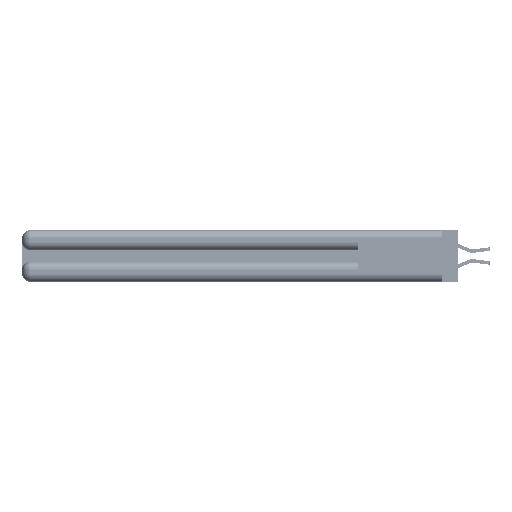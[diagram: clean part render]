
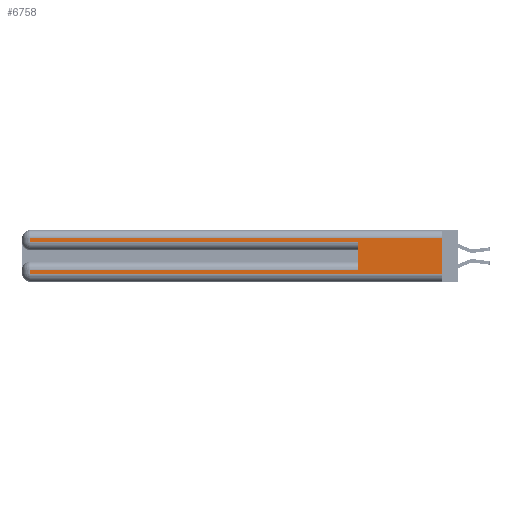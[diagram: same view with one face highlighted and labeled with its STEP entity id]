
A CAD part, left-side view. The second image highlights one B-rep face of the part: STEP entity #6758.
In plain terms, the highlighted planar face has unit normal (-1, 0, 0).
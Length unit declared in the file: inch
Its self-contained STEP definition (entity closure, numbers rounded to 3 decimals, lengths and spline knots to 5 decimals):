
#1256 = LINE ( 'NONE', #49349, #53000 ) ;
#1796 = VERTEX_POINT ( 'NONE', #38416 ) ;
#1999 = CARTESIAN_POINT ( 'NONE',  ( 0., 0., 0.37 ) ) ;
#2927 = ORIENTED_EDGE ( 'NONE', *, *, #8571, .T. ) ;
#2990 = EDGE_CURVE ( 'NONE', #17240, #33682, #16627, .T. ) ;
#3101 = VECTOR ( 'NONE', #3349, 39.37008 ) ;
#3349 = DIRECTION ( 'NONE',  ( 0., -1., 0. ) ) ;
#3509 = CARTESIAN_POINT ( 'NONE',  ( 0., 0., 0.285 ) ) ;
#3828 = DIRECTION ( 'NONE',  ( 0., 1., 0. ) ) ;
#4285 = LINE ( 'NONE', #1999, #22277 ) ;
#6686 = DIRECTION ( 'NONE',  ( 0., 0., -1. ) ) ;
#6758 = ADVANCED_FACE ( 'NONE', ( #38635 ), #25982, .F. ) ;
#7162 = CARTESIAN_POINT ( 'NONE',  ( 0., 0., 0.31 ) ) ;
#8322 = EDGE_CURVE ( 'NONE', #31892, #1796, #20441, .T. ) ;
#8571 = EDGE_CURVE ( 'NONE', #39538, #28233, #33320, .T. ) ;
#9520 = VECTOR ( 'NONE', #6686, 39.37008 ) ;
#10429 = CARTESIAN_POINT ( 'NONE',  ( 0., 2.94, 0.31 ) ) ;
#10934 = EDGE_CURVE ( 'NONE', #31908, #1796, #4285, .T. ) ;
#11728 = DIRECTION ( 'NONE',  ( 0., -1., 0. ) ) ;
#12403 = ORIENTED_EDGE ( 'NONE', *, *, #24803, .T. ) ;
#13508 = CARTESIAN_POINT ( 'NONE',  ( 0., 0., 0.37 ) ) ;
#14196 = DIRECTION ( 'NONE',  ( 0., 0., -1. ) ) ;
#16627 = LINE ( 'NONE', #38721, #38555 ) ;
#17240 = VERTEX_POINT ( 'NONE', #43411 ) ;
#18455 = EDGE_CURVE ( 'NONE', #31908, #39538, #1256, .T. ) ;
#19855 = CARTESIAN_POINT ( 'NONE',  ( 0., 0., 0.06 ) ) ;
#20441 = LINE ( 'NONE', #19855, #3101 ) ;
#20794 = CARTESIAN_POINT ( 'NONE',  ( 0., 2.94, 0.285 ) ) ;
#21279 = VECTOR ( 'NONE', #11728, 39.37008 ) ;
#21494 = DIRECTION ( 'NONE',  ( 0., 0., 1. ) ) ;
#22235 = AXIS2_PLACEMENT_3D ( 'NONE', #13508, #42412, #46280 ) ;
#22277 = VECTOR ( 'NONE', #14196, 39.37008 ) ;
#23624 = CARTESIAN_POINT ( 'NONE',  ( 0., 2.94, 0.37 ) ) ;
#23753 = VERTEX_POINT ( 'NONE', #45072 ) ;
#24803 = EDGE_CURVE ( 'NONE', #33682, #31892, #35378, .T. ) ;
#25114 = ORIENTED_EDGE ( 'NONE', *, *, #2990, .T. ) ;
#25233 = LINE ( 'NONE', #3509, #21279 ) ;
#25982 = PLANE ( 'NONE',  #22235 ) ;
#26838 = ORIENTED_EDGE ( 'NONE', *, *, #38016, .F. ) ;
#27167 = LINE ( 'NONE', #29460, #42038 ) ;
#28233 = VERTEX_POINT ( 'NONE', #20794 ) ;
#29460 = CARTESIAN_POINT ( 'NONE',  ( 0., 0.6, 0.145 ) ) ;
#31892 = VERTEX_POINT ( 'NONE', #52758 ) ;
#31908 = VERTEX_POINT ( 'NONE', #7162 ) ;
#33320 = LINE ( 'NONE', #23624, #9520 ) ;
#33519 = ORIENTED_EDGE ( 'NONE', *, *, #8322, .T. ) ;
#33682 = VERTEX_POINT ( 'NONE', #35364 ) ;
#35171 = CARTESIAN_POINT ( 'NONE',  ( 0., 2.94, 0.37 ) ) ;
#35364 = CARTESIAN_POINT ( 'NONE',  ( 0., 2.94, 0.085 ) ) ;
#35378 = LINE ( 'NONE', #35171, #38596 ) ;
#35699 = ORIENTED_EDGE ( 'NONE', *, *, #10934, .F. ) ;
#38016 = EDGE_CURVE ( 'NONE', #17240, #23753, #27167, .T. ) ;
#38258 = ORIENTED_EDGE ( 'NONE', *, *, #18455, .T. ) ;
#38358 = DIRECTION ( 'NONE',  ( 0., 1., 0. ) ) ;
#38397 = EDGE_CURVE ( 'NONE', #28233, #23753, #25233, .T. ) ;
#38416 = CARTESIAN_POINT ( 'NONE',  ( 0., 0., 0.06 ) ) ;
#38555 = VECTOR ( 'NONE', #38358, 39.37008 ) ;
#38596 = VECTOR ( 'NONE', #51197, 39.37008 ) ;
#38635 = FACE_OUTER_BOUND ( 'NONE', #46089, .T. ) ;
#38721 = CARTESIAN_POINT ( 'NONE',  ( 0., 0., 0.085 ) ) ;
#39538 = VERTEX_POINT ( 'NONE', #10429 ) ;
#42038 = VECTOR ( 'NONE', #21494, 39.37008 ) ;
#42412 = DIRECTION ( 'NONE',  ( 1., 0., 0. ) ) ;
#43411 = CARTESIAN_POINT ( 'NONE',  ( 0., 0.6, 0.085 ) ) ;
#44473 = ORIENTED_EDGE ( 'NONE', *, *, #38397, .T. ) ;
#45072 = CARTESIAN_POINT ( 'NONE',  ( 0., 0.6, 0.285 ) ) ;
#46089 = EDGE_LOOP ( 'NONE', ( #35699, #38258, #2927, #44473, #26838, #25114, #12403, #33519 ) ) ;
#46280 = DIRECTION ( 'NONE',  ( 0., 0., -1. ) ) ;
#49349 = CARTESIAN_POINT ( 'NONE',  ( 0., 0., 0.31 ) ) ;
#51197 = DIRECTION ( 'NONE',  ( 0., 0., -1. ) ) ;
#52758 = CARTESIAN_POINT ( 'NONE',  ( 0., 2.94, 0.06 ) ) ;
#53000 = VECTOR ( 'NONE', #3828, 39.37008 ) ;
